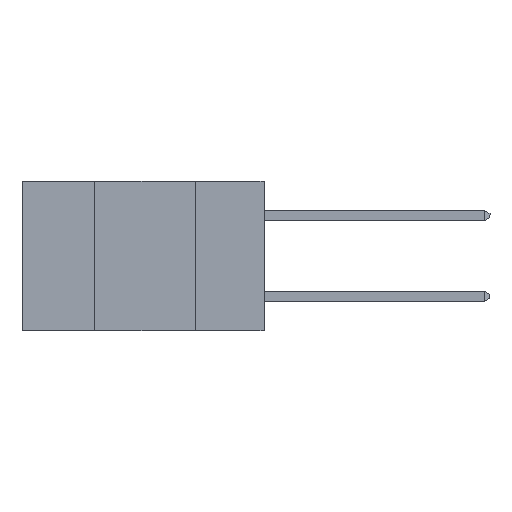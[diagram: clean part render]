
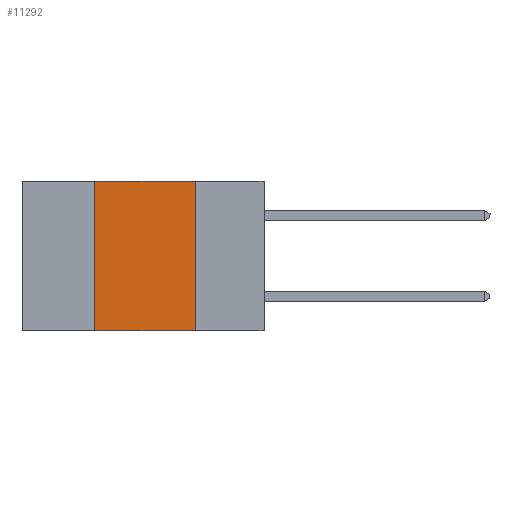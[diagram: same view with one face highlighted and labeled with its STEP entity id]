
A CAD part, left-side view. The second image highlights one B-rep face of the part: STEP entity #11292.
In plain terms, the highlighted planar face has unit normal (-1, 0, 0).
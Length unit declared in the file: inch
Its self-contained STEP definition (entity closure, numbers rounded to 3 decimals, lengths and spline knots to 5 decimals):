
#591 = VERTEX_POINT ( 'NONE', #4995 ) ;
#829 = VECTOR ( 'NONE', #9876, 39.37008 ) ;
#899 = CARTESIAN_POINT ( 'NONE',  ( 0., 0.6, -0.37 ) ) ;
#2017 = DIRECTION ( 'NONE',  ( 1., 0., 0. ) ) ;
#3152 = VERTEX_POINT ( 'NONE', #11176 ) ;
#3354 = VECTOR ( 'NONE', #4265, 39.37008 ) ;
#3852 = EDGE_CURVE ( 'NONE', #11288, #3152, #10732, .T. ) ;
#4052 = EDGE_CURVE ( 'NONE', #7200, #11288, #6108, .T. ) ;
#4265 = DIRECTION ( 'NONE',  ( 0., 0., -1. ) ) ;
#4385 = ORIENTED_EDGE ( 'NONE', *, *, #4052, .F. ) ;
#4396 = CARTESIAN_POINT ( 'NONE',  ( 0., 0.17, 0. ) ) ;
#4806 = LINE ( 'NONE', #899, #9580 ) ;
#4976 = CARTESIAN_POINT ( 'NONE',  ( 0., 0.6, 0. ) ) ;
#4995 = CARTESIAN_POINT ( 'NONE',  ( 0., 0.42, -0.37 ) ) ;
#6108 = LINE ( 'NONE', #6340, #829 ) ;
#6340 = CARTESIAN_POINT ( 'NONE',  ( 0., 0.6, 0. ) ) ;
#6491 = VECTOR ( 'NONE', #12211, 39.37008 ) ;
#6715 = AXIS2_PLACEMENT_3D ( 'NONE', #4976, #2017, #8812 ) ;
#6825 = DIRECTION ( 'NONE',  ( 0., -1., 0. ) ) ;
#6885 = PLANE ( 'NONE',  #6715 ) ;
#7058 = ORIENTED_EDGE ( 'NONE', *, *, #11857, .T. ) ;
#7200 = VERTEX_POINT ( 'NONE', #8917 ) ;
#7432 = CARTESIAN_POINT ( 'NONE',  ( 0., 0.42, 0. ) ) ;
#8140 = EDGE_LOOP ( 'NONE', ( #11581, #4385, #8580, #7058 ) ) ;
#8580 = ORIENTED_EDGE ( 'NONE', *, *, #10469, .F. ) ;
#8812 = DIRECTION ( 'NONE',  ( 0., 0., -1. ) ) ;
#8917 = CARTESIAN_POINT ( 'NONE',  ( 0., 0.42, 0. ) ) ;
#8995 = LINE ( 'NONE', #7432, #6491 ) ;
#9447 = FACE_OUTER_BOUND ( 'NONE', #8140, .T. ) ;
#9580 = VECTOR ( 'NONE', #6825, 39.37008 ) ;
#9876 = DIRECTION ( 'NONE',  ( 0., -1., 0. ) ) ;
#10469 = EDGE_CURVE ( 'NONE', #591, #7200, #8995, .T. ) ;
#10732 = LINE ( 'NONE', #4396, #3354 ) ;
#11176 = CARTESIAN_POINT ( 'NONE',  ( 0., 0.17, -0.37 ) ) ;
#11288 = VERTEX_POINT ( 'NONE', #11655 ) ;
#11292 = ADVANCED_FACE ( 'NONE', ( #9447 ), #6885, .F. ) ;
#11581 = ORIENTED_EDGE ( 'NONE', *, *, #3852, .F. ) ;
#11655 = CARTESIAN_POINT ( 'NONE',  ( 0., 0.17, 0. ) ) ;
#11857 = EDGE_CURVE ( 'NONE', #591, #3152, #4806, .T. ) ;
#12211 = DIRECTION ( 'NONE',  ( 0., 0., 1. ) ) ;
